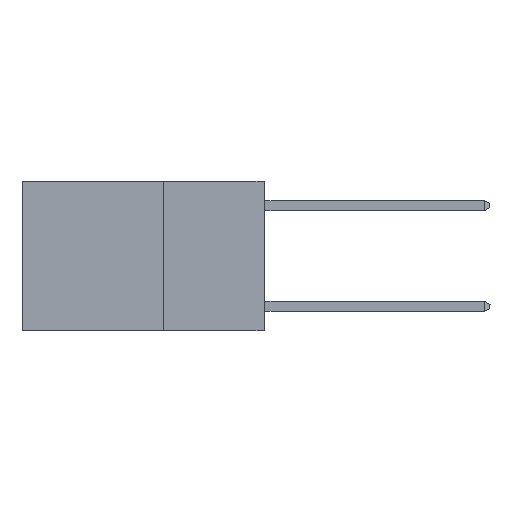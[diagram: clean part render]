
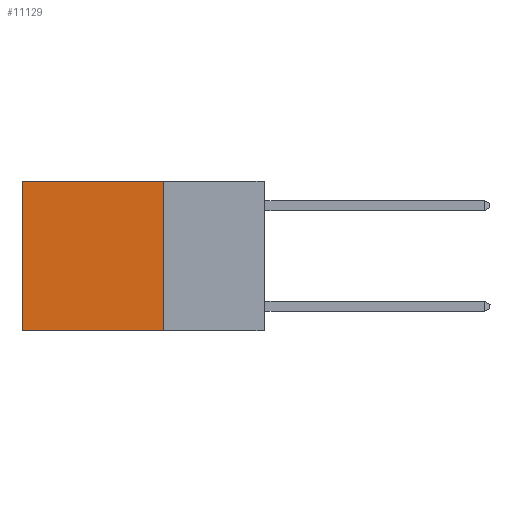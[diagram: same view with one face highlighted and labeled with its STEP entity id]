
A CAD part, left-side view. The second image highlights one B-rep face of the part: STEP entity #11129.
In plain terms, the highlighted planar face has unit normal (-1, 0, 0).
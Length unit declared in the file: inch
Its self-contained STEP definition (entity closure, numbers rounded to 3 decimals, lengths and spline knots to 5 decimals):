
#858 = DIRECTION ( 'NONE',  ( 1., 0., 0. ) ) ;
#1075 = VERTEX_POINT ( 'NONE', #3081 ) ;
#1877 = LINE ( 'NONE', #8979, #10828 ) ;
#2480 = EDGE_CURVE ( 'NONE', #1075, #7793, #15192, .T. ) ;
#3081 = CARTESIAN_POINT ( 'NONE',  ( 0.2625, 0.25, 0. ) ) ;
#3753 = ORIENTED_EDGE ( 'NONE', *, *, #13319, .T. ) ;
#4857 = ORIENTED_EDGE ( 'NONE', *, *, #6870, .T. ) ;
#5124 = PLANE ( 'NONE',  #7606 ) ;
#6870 = EDGE_CURVE ( 'NONE', #1075, #13046, #13119, .T. ) ;
#6875 = FACE_OUTER_BOUND ( 'NONE', #10689, .T. ) ;
#7202 = CARTESIAN_POINT ( 'NONE',  ( 0.2625, 0.25, 0. ) ) ;
#7606 = AXIS2_PLACEMENT_3D ( 'NONE', #8135, #858, #18329 ) ;
#7703 = DIRECTION ( 'NONE',  ( 0., 0., -1. ) ) ;
#7793 = VERTEX_POINT ( 'NONE', #9088 ) ;
#8135 = CARTESIAN_POINT ( 'NONE',  ( 0.2625, 0.25, 0. ) ) ;
#8216 = VECTOR ( 'NONE', #10046, 39.37008 ) ;
#8916 = LINE ( 'NONE', #9172, #16125 ) ;
#8952 = CARTESIAN_POINT ( 'NONE',  ( 0.2625, 0.25, 0. ) ) ;
#8979 = CARTESIAN_POINT ( 'NONE',  ( 0.2625, 0.6, 0. ) ) ;
#9088 = CARTESIAN_POINT ( 'NONE',  ( 0.2625, 0.25, -0.37 ) ) ;
#9140 = DIRECTION ( 'NONE',  ( 0., 0., -1. ) ) ;
#9172 = CARTESIAN_POINT ( 'NONE',  ( 0.2625, 0.25, -0.37 ) ) ;
#9537 = CARTESIAN_POINT ( 'NONE',  ( 0.2625, 0.6, 0. ) ) ;
#9800 = VECTOR ( 'NONE', #9140, 39.37008 ) ;
#10046 = DIRECTION ( 'NONE',  ( 0., 1., 0. ) ) ;
#10689 = EDGE_LOOP ( 'NONE', ( #3753, #11682, #18143, #4857 ) ) ;
#10828 = VECTOR ( 'NONE', #7703, 39.37008 ) ;
#11129 = ADVANCED_FACE ( 'NONE', ( #6875 ), #5124, .F. ) ;
#11682 = ORIENTED_EDGE ( 'NONE', *, *, #13460, .F. ) ;
#12891 = CARTESIAN_POINT ( 'NONE',  ( 0.2625, 0.6, -0.37 ) ) ;
#13046 = VERTEX_POINT ( 'NONE', #9537 ) ;
#13119 = LINE ( 'NONE', #7202, #8216 ) ;
#13319 = EDGE_CURVE ( 'NONE', #13046, #15061, #1877, .T. ) ;
#13460 = EDGE_CURVE ( 'NONE', #7793, #15061, #8916, .T. ) ;
#15061 = VERTEX_POINT ( 'NONE', #12891 ) ;
#15192 = LINE ( 'NONE', #8952, #9800 ) ;
#16125 = VECTOR ( 'NONE', #17792, 39.37008 ) ;
#17792 = DIRECTION ( 'NONE',  ( 0., 1., 0. ) ) ;
#18143 = ORIENTED_EDGE ( 'NONE', *, *, #2480, .F. ) ;
#18329 = DIRECTION ( 'NONE',  ( 0., 0., -1. ) ) ;
